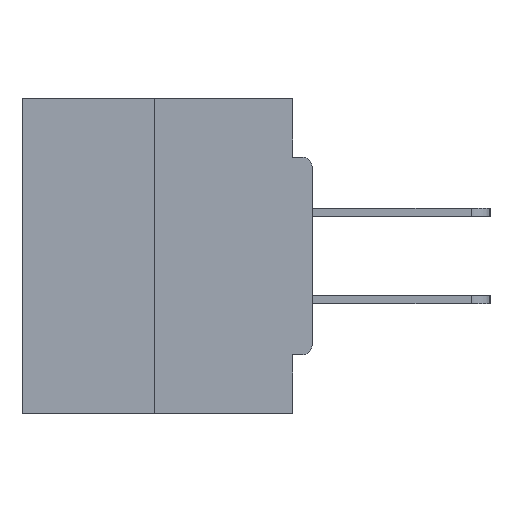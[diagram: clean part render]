
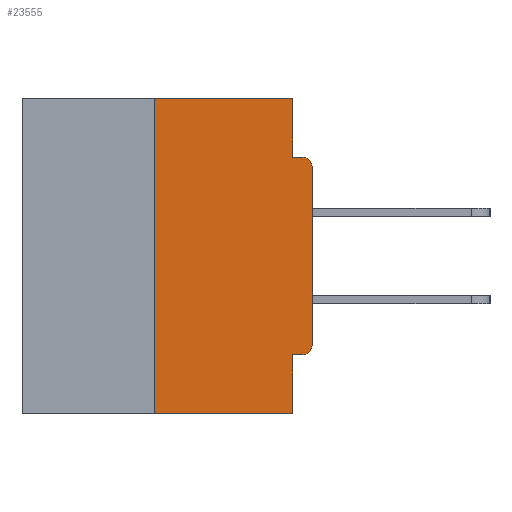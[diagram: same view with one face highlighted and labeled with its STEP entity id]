
A CAD part, left-side view. The second image highlights one B-rep face of the part: STEP entity #23555.
In plain terms, the highlighted planar face has unit normal (-1, 0, 0).
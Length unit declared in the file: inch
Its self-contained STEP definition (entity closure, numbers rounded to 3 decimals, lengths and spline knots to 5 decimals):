
#31 = ORIENTED_EDGE ( 'NONE', *, *, #14716, .F. ) ;
#584 = DIRECTION ( 'NONE',  ( 0., 0., -1. ) ) ;
#798 = CIRCLE ( 'NONE', #11347, 0.015 ) ;
#1091 = ORIENTED_EDGE ( 'NONE', *, *, #28349, .T. ) ;
#2673 = DIRECTION ( 'NONE',  ( 0., 0., -1. ) ) ;
#3264 = VECTOR ( 'NONE', #16760, 39.37008 ) ;
#3541 = CARTESIAN_POINT ( 'NONE',  ( 0., 0.031, -0.5 ) ) ;
#3878 = DIRECTION ( 'NONE',  ( -1., 0., 0. ) ) ;
#4355 = ORIENTED_EDGE ( 'NONE', *, *, #4992, .F. ) ;
#4605 = CARTESIAN_POINT ( 'NONE',  ( 0., 0.25, 0. ) ) ;
#4624 = CARTESIAN_POINT ( 'NONE',  ( 0., 0.25, -0.5 ) ) ;
#4992 = EDGE_CURVE ( 'NONE', #33054, #13237, #8533, .T. ) ;
#5130 = VECTOR ( 'NONE', #17529, 39.37008 ) ;
#5465 = DIRECTION ( 'NONE',  ( 0., 1., 0. ) ) ;
#5746 = DIRECTION ( 'NONE',  ( 1., 0., 0. ) ) ;
#6205 = CARTESIAN_POINT ( 'NONE',  ( 0., 0.46, 0. ) ) ;
#6218 = EDGE_CURVE ( 'NONE', #13692, #25525, #28538, .T. ) ;
#6288 = ORIENTED_EDGE ( 'NONE', *, *, #33183, .T. ) ;
#7681 = VERTEX_POINT ( 'NONE', #21815 ) ;
#8133 = ORIENTED_EDGE ( 'NONE', *, *, #11476, .F. ) ;
#8533 = LINE ( 'NONE', #21225, #14513 ) ;
#8783 = PLANE ( 'NONE',  #25618 ) ;
#9175 = VECTOR ( 'NONE', #15778, 39.37008 ) ;
#9516 = CARTESIAN_POINT ( 'NONE',  ( 0., 0.46, -0.5 ) ) ;
#9682 = CARTESIAN_POINT ( 'NONE',  ( 0., 0.015, -0.0935 ) ) ;
#10141 = CARTESIAN_POINT ( 'NONE',  ( 0., 0.031, 0. ) ) ;
#11347 = AXIS2_PLACEMENT_3D ( 'NONE', #32253, #3878, #14913 ) ;
#11419 = VERTEX_POINT ( 'NONE', #4605 ) ;
#11476 = EDGE_CURVE ( 'NONE', #24248, #14571, #32947, .T. ) ;
#11542 = CARTESIAN_POINT ( 'NONE',  ( 0., 0.031, 0. ) ) ;
#11854 = VERTEX_POINT ( 'NONE', #11542 ) ;
#12271 = DIRECTION ( 'NONE',  ( 0., 0., -1. ) ) ;
#12316 = ORIENTED_EDGE ( 'NONE', *, *, #26220, .T. ) ;
#12336 = DIRECTION ( 'NONE',  ( 0., 0., 1. ) ) ;
#13237 = VERTEX_POINT ( 'NONE', #29785 ) ;
#13501 = EDGE_LOOP ( 'NONE', ( #32509, #17535, #30652, #24564, #4355, #1091, #12316, #6288, #8133, #31 ) ) ;
#13692 = VERTEX_POINT ( 'NONE', #4624 ) ;
#14513 = VECTOR ( 'NONE', #5465, 39.37008 ) ;
#14571 = VERTEX_POINT ( 'NONE', #9682 ) ;
#14716 = EDGE_CURVE ( 'NONE', #11854, #24248, #29822, .T. ) ;
#14913 = DIRECTION ( 'NONE',  ( 0., 0., -1. ) ) ;
#15778 = DIRECTION ( 'NONE',  ( 0., 0., 1. ) ) ;
#16389 = DIRECTION ( 'NONE',  ( 0., 0., -1. ) ) ;
#16760 = DIRECTION ( 'NONE',  ( 0., -1., 0. ) ) ;
#17354 = CARTESIAN_POINT ( 'NONE',  ( 0., 0., 0. ) ) ;
#17529 = DIRECTION ( 'NONE',  ( 0., -1., 0. ) ) ;
#17535 = ORIENTED_EDGE ( 'NONE', *, *, #29247, .F. ) ;
#17548 = CARTESIAN_POINT ( 'NONE',  ( 0., 0., -0.1085 ) ) ;
#19183 = VECTOR ( 'NONE', #16389, 39.37008 ) ;
#19907 = DIRECTION ( 'NONE',  ( 0., -1., 0. ) ) ;
#20794 = CARTESIAN_POINT ( 'NONE',  ( 0., 0.015, -0.1085 ) ) ;
#21225 = CARTESIAN_POINT ( 'NONE',  ( 0., 0., -0.4065 ) ) ;
#21815 = CARTESIAN_POINT ( 'NONE',  ( 0., 0., -0.3915 ) ) ;
#21908 = CARTESIAN_POINT ( 'NONE',  ( 0., 0.015, -0.4065 ) ) ;
#21945 = EDGE_CURVE ( 'NONE', #13237, #25525, #26844, .T. ) ;
#23555 = ADVANCED_FACE ( 'NONE', ( #25563 ), #8783, .F. ) ;
#24248 = VERTEX_POINT ( 'NONE', #28634 ) ;
#24564 = ORIENTED_EDGE ( 'NONE', *, *, #21945, .F. ) ;
#24572 = VECTOR ( 'NONE', #12336, 39.37008 ) ;
#25470 = AXIS2_PLACEMENT_3D ( 'NONE', #20794, #25963, #2673 ) ;
#25525 = VERTEX_POINT ( 'NONE', #25539 ) ;
#25539 = CARTESIAN_POINT ( 'NONE',  ( 0., 0.031, -0.5 ) ) ;
#25563 = FACE_OUTER_BOUND ( 'NONE', #13501, .T. ) ;
#25615 = CARTESIAN_POINT ( 'NONE',  ( 0., 0.46, 0. ) ) ;
#25618 = AXIS2_PLACEMENT_3D ( 'NONE', #6205, #5746, #584 ) ;
#25963 = DIRECTION ( 'NONE',  ( -1., 0., 0. ) ) ;
#26220 = EDGE_CURVE ( 'NONE', #7681, #27925, #31421, .T. ) ;
#26226 = CIRCLE ( 'NONE', #25470, 0.015 ) ;
#26394 = LINE ( 'NONE', #30899, #9175 ) ;
#26844 = LINE ( 'NONE', #3541, #19183 ) ;
#26998 = VECTOR ( 'NONE', #12271, 39.37008 ) ;
#27925 = VERTEX_POINT ( 'NONE', #17548 ) ;
#28349 = EDGE_CURVE ( 'NONE', #33054, #7681, #798, .T. ) ;
#28538 = LINE ( 'NONE', #9516, #3264 ) ;
#28634 = CARTESIAN_POINT ( 'NONE',  ( 0., 0.031, -0.0935 ) ) ;
#29247 = EDGE_CURVE ( 'NONE', #13692, #11419, #26394, .T. ) ;
#29744 = EDGE_CURVE ( 'NONE', #11419, #11854, #33211, .T. ) ;
#29785 = CARTESIAN_POINT ( 'NONE',  ( 0., 0.031, -0.4065 ) ) ;
#29822 = LINE ( 'NONE', #10141, #26998 ) ;
#30187 = CARTESIAN_POINT ( 'NONE',  ( 0., 0., -0.0935 ) ) ;
#30546 = VECTOR ( 'NONE', #19907, 39.37008 ) ;
#30652 = ORIENTED_EDGE ( 'NONE', *, *, #6218, .T. ) ;
#30899 = CARTESIAN_POINT ( 'NONE',  ( 0., 0.25, 0. ) ) ;
#31421 = LINE ( 'NONE', #17354, #24572 ) ;
#32253 = CARTESIAN_POINT ( 'NONE',  ( 0., 0.015, -0.3915 ) ) ;
#32509 = ORIENTED_EDGE ( 'NONE', *, *, #29744, .F. ) ;
#32947 = LINE ( 'NONE', #30187, #30546 ) ;
#33054 = VERTEX_POINT ( 'NONE', #21908 ) ;
#33183 = EDGE_CURVE ( 'NONE', #27925, #14571, #26226, .T. ) ;
#33211 = LINE ( 'NONE', #25615, #5130 ) ;
